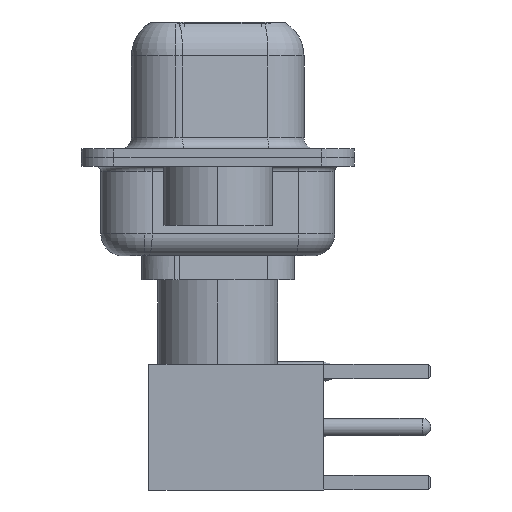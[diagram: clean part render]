
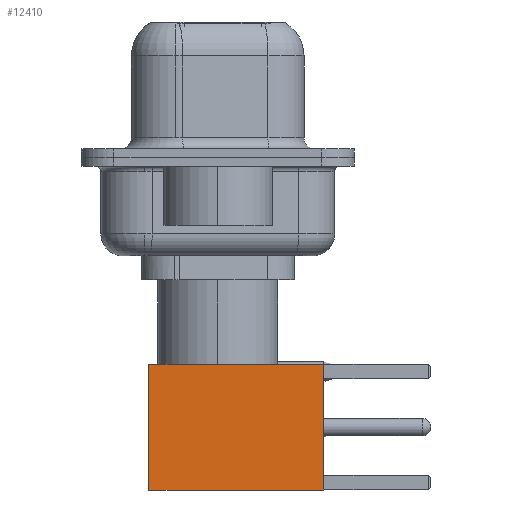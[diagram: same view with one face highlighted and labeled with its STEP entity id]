
A CAD part, left-side view. The second image highlights one B-rep face of the part: STEP entity #12410.
In plain terms, the highlighted face is planar.
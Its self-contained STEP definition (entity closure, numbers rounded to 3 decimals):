
#240 = LINE ( 'NONE', #14289, #2058 ) ;
#317 = EDGE_CURVE ( 'NONE', #22536, #6636, #240, .T. ) ;
#1033 = CARTESIAN_POINT ( 'NONE',  ( 0., 2.875, 0. ) ) ;
#1532 = CARTESIAN_POINT ( 'NONE',  ( -2.875, 2.875, 8. ) ) ;
#2058 = VECTOR ( 'NONE', #18089, 1000. ) ;
#3002 = LINE ( 'NONE', #1033, #12651 ) ;
#3654 = LINE ( 'NONE', #15836, #12095 ) ;
#3832 = DIRECTION ( 'NONE',  ( 0., 0., -1. ) ) ;
#4417 = CARTESIAN_POINT ( 'NONE',  ( 2.875, 2.875, 8. ) ) ;
#5185 = AXIS2_PLACEMENT_3D ( 'NONE', #15003, #20075, #16607 ) ;
#5792 = FACE_OUTER_BOUND ( 'NONE', #16787, .T. ) ;
#5855 = CARTESIAN_POINT ( 'NONE',  ( -2.875, 2.875, 0. ) ) ;
#6636 = VERTEX_POINT ( 'NONE', #5855 ) ;
#8136 = VECTOR ( 'NONE', #3832, 1000. ) ;
#8241 = ORIENTED_EDGE ( 'NONE', *, *, #317, .F. ) ;
#10810 = EDGE_CURVE ( 'NONE', #12388, #22536, #3654, .T. ) ;
#11106 = CARTESIAN_POINT ( 'NONE',  ( 2.875, 2.875, 0. ) ) ;
#12095 = VECTOR ( 'NONE', #12619, 1000. ) ;
#12388 = VERTEX_POINT ( 'NONE', #4417 ) ;
#12410 = ADVANCED_FACE ( 'NONE', ( #5792 ), #13054, .T. ) ;
#12614 = EDGE_CURVE ( 'NONE', #12388, #20768, #19586, .T. ) ;
#12619 = DIRECTION ( 'NONE',  ( -1., 0., 0. ) ) ;
#12651 = VECTOR ( 'NONE', #15088, 1000. ) ;
#13054 = PLANE ( 'NONE',  #5185 ) ;
#13885 = ORIENTED_EDGE ( 'NONE', *, *, #16633, .T. ) ;
#14289 = CARTESIAN_POINT ( 'NONE',  ( -2.875, 2.875, 0. ) ) ;
#15003 = CARTESIAN_POINT ( 'NONE',  ( 2.875, 2.875, 0. ) ) ;
#15088 = DIRECTION ( 'NONE',  ( -1., 0., 0. ) ) ;
#15836 = CARTESIAN_POINT ( 'NONE',  ( 0., 2.875, 8. ) ) ;
#16607 = DIRECTION ( 'NONE',  ( 0., 0., 1. ) ) ;
#16633 = EDGE_CURVE ( 'NONE', #20768, #6636, #3002, .T. ) ;
#16787 = EDGE_LOOP ( 'NONE', ( #22425, #13885, #8241, #21223 ) ) ;
#18089 = DIRECTION ( 'NONE',  ( 0., 0., -1. ) ) ;
#19586 = LINE ( 'NONE', #22713, #8136 ) ;
#20075 = DIRECTION ( 'NONE',  ( 0., 1., 0. ) ) ;
#20768 = VERTEX_POINT ( 'NONE', #11106 ) ;
#21223 = ORIENTED_EDGE ( 'NONE', *, *, #10810, .F. ) ;
#22425 = ORIENTED_EDGE ( 'NONE', *, *, #12614, .T. ) ;
#22536 = VERTEX_POINT ( 'NONE', #1532 ) ;
#22713 = CARTESIAN_POINT ( 'NONE',  ( 2.875, 2.875, 0. ) ) ;
